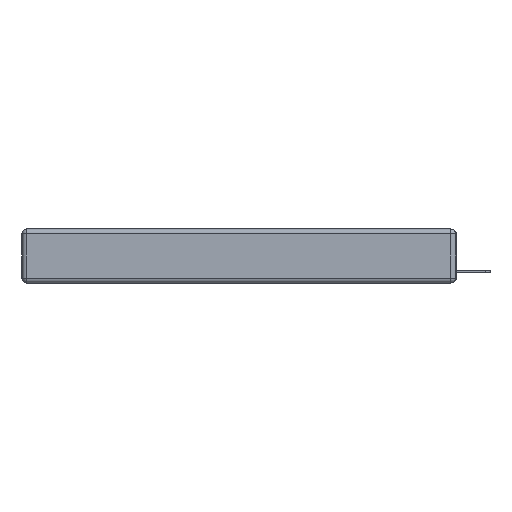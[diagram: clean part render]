
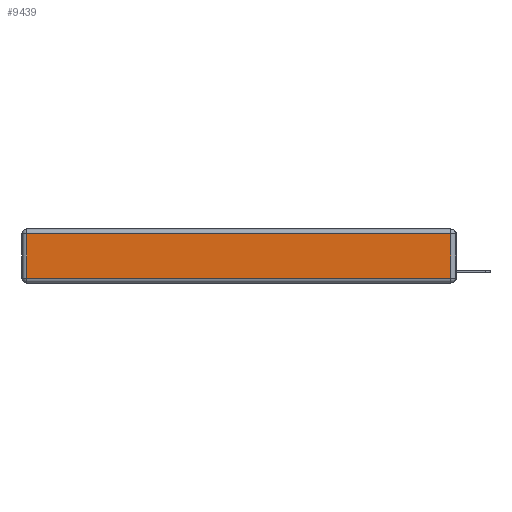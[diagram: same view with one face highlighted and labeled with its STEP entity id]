
A CAD part, left-side view. The second image highlights one B-rep face of the part: STEP entity #9439.
In plain terms, the highlighted planar face has unit normal (-1, 0, 0).
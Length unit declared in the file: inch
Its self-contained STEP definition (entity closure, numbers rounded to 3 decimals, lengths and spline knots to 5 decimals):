
#747 = CARTESIAN_POINT ( 'NONE',  ( 0., 2.72, -0.313 ) ) ;
#863 = DIRECTION ( 'NONE',  ( 0., -1., 0. ) ) ;
#2045 = VERTEX_POINT ( 'NONE', #747 ) ;
#4097 = LINE ( 'NONE', #4841, #7047 ) ;
#4139 = DIRECTION ( 'NONE',  ( 0., 0., 1. ) ) ;
#4210 = AXIS2_PLACEMENT_3D ( 'NONE', #13646, #15637, #4139 ) ;
#4841 = CARTESIAN_POINT ( 'NONE',  ( 0., 2.72, -0.343 ) ) ;
#5057 = ORIENTED_EDGE ( 'NONE', *, *, #11709, .T. ) ;
#5350 = VECTOR ( 'NONE', #863, 39.37008 ) ;
#6249 = LINE ( 'NONE', #18548, #12704 ) ;
#7047 = VECTOR ( 'NONE', #19037, 39.37008 ) ;
#7763 = DIRECTION ( 'NONE',  ( 0., 1., 0. ) ) ;
#9439 = ADVANCED_FACE ( 'NONE', ( #13047 ), #10441, .T. ) ;
#9704 = ORIENTED_EDGE ( 'NONE', *, *, #18677, .T. ) ;
#10184 = EDGE_CURVE ( 'NONE', #13503, #2045, #4097, .T. ) ;
#10256 = VECTOR ( 'NONE', #7763, 39.37008 ) ;
#10441 = PLANE ( 'NONE',  #4210 ) ;
#10762 = VERTEX_POINT ( 'NONE', #19461 ) ;
#10842 = CARTESIAN_POINT ( 'NONE',  ( 0., 2.75, -0.03 ) ) ;
#11709 = EDGE_CURVE ( 'NONE', #17444, #10762, #6249, .T. ) ;
#11992 = CARTESIAN_POINT ( 'NONE',  ( 0., 0.03, -0.313 ) ) ;
#12704 = VECTOR ( 'NONE', #18758, 39.37008 ) ;
#12843 = CARTESIAN_POINT ( 'NONE',  ( 0., 2.72, -0.03 ) ) ;
#13047 = FACE_OUTER_BOUND ( 'NONE', #16223, .T. ) ;
#13503 = VERTEX_POINT ( 'NONE', #12843 ) ;
#13646 = CARTESIAN_POINT ( 'NONE',  ( 0., 0., -0.343 ) ) ;
#14497 = EDGE_CURVE ( 'NONE', #10762, #13503, #16666, .T. ) ;
#14986 = ORIENTED_EDGE ( 'NONE', *, *, #14497, .T. ) ;
#15637 = DIRECTION ( 'NONE',  ( -1., 0., 0. ) ) ;
#16223 = EDGE_LOOP ( 'NONE', ( #9704, #5057, #14986, #19090 ) ) ;
#16666 = LINE ( 'NONE', #10842, #10256 ) ;
#17444 = VERTEX_POINT ( 'NONE', #11992 ) ;
#17984 = LINE ( 'NONE', #19931, #5350 ) ;
#18548 = CARTESIAN_POINT ( 'NONE',  ( 0., 0.03, -0.343 ) ) ;
#18677 = EDGE_CURVE ( 'NONE', #2045, #17444, #17984, .T. ) ;
#18758 = DIRECTION ( 'NONE',  ( 0., 0., 1. ) ) ;
#19037 = DIRECTION ( 'NONE',  ( 0., 0., -1. ) ) ;
#19090 = ORIENTED_EDGE ( 'NONE', *, *, #10184, .T. ) ;
#19461 = CARTESIAN_POINT ( 'NONE',  ( 0., 0.03, -0.03 ) ) ;
#19931 = CARTESIAN_POINT ( 'NONE',  ( 0., 0., -0.313 ) ) ;
